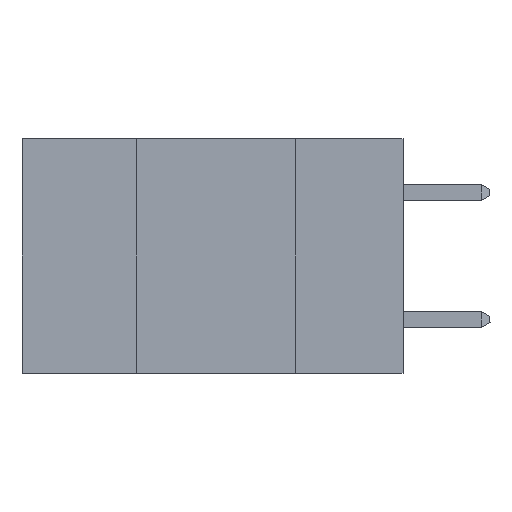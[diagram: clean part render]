
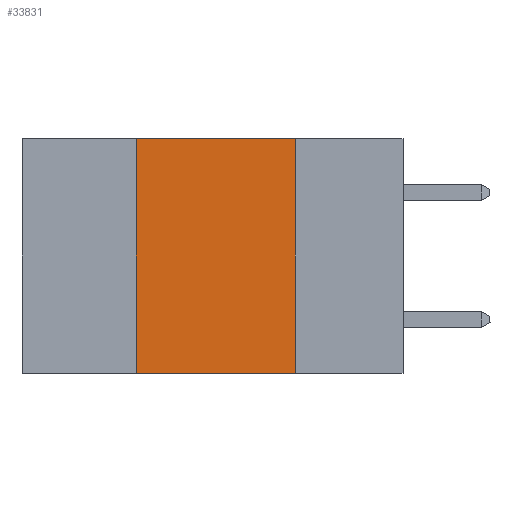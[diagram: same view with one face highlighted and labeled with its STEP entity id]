
A CAD part, left-side view. The second image highlights one B-rep face of the part: STEP entity #33831.
In plain terms, the highlighted planar face has unit normal (-1, 0, 0).
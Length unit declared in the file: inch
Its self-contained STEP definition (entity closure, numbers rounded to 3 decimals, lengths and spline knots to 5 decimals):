
#462 = VERTEX_POINT ( 'NONE', #35231 ) ;
#1846 = VECTOR ( 'NONE', #3232, 39.37008 ) ;
#3232 = DIRECTION ( 'NONE',  ( 0., 0., -1. ) ) ;
#3830 = CARTESIAN_POINT ( 'NONE',  ( 0., 0.17, 0. ) ) ;
#4133 = EDGE_CURVE ( 'NONE', #462, #19122, #25147, .T. ) ;
#5890 = CARTESIAN_POINT ( 'NONE',  ( 0., 0.42, -0.37 ) ) ;
#7984 = CARTESIAN_POINT ( 'NONE',  ( 0., 0.6, 0. ) ) ;
#8055 = EDGE_LOOP ( 'NONE', ( #14364, #28024, #12784, #22752 ) ) ;
#9670 = CARTESIAN_POINT ( 'NONE',  ( 0., 0.42, 0. ) ) ;
#11705 = LINE ( 'NONE', #24902, #14326 ) ;
#12784 = ORIENTED_EDGE ( 'NONE', *, *, #13157, .F. ) ;
#13157 = EDGE_CURVE ( 'NONE', #30707, #26317, #32740, .T. ) ;
#13160 = DIRECTION ( 'NONE',  ( 0., -1., 0. ) ) ;
#14326 = VECTOR ( 'NONE', #19007, 39.37008 ) ;
#14364 = ORIENTED_EDGE ( 'NONE', *, *, #4133, .F. ) ;
#16436 = DIRECTION ( 'NONE',  ( 0., 0., -1. ) ) ;
#16932 = VECTOR ( 'NONE', #34875, 39.37008 ) ;
#17574 = CARTESIAN_POINT ( 'NONE',  ( 0., 0.42, 0. ) ) ;
#19007 = DIRECTION ( 'NONE',  ( 0., -1., 0. ) ) ;
#19122 = VERTEX_POINT ( 'NONE', #19761 ) ;
#19761 = CARTESIAN_POINT ( 'NONE',  ( 0., 0.17, -0.37 ) ) ;
#21827 = AXIS2_PLACEMENT_3D ( 'NONE', #7984, #27585, #16436 ) ;
#22752 = ORIENTED_EDGE ( 'NONE', *, *, #34314, .T. ) ;
#24813 = PLANE ( 'NONE',  #21827 ) ;
#24902 = CARTESIAN_POINT ( 'NONE',  ( 0., 0.6, -0.37 ) ) ;
#25147 = LINE ( 'NONE', #3830, #1846 ) ;
#26317 = VERTEX_POINT ( 'NONE', #17574 ) ;
#27059 = LINE ( 'NONE', #35872, #34124 ) ;
#27585 = DIRECTION ( 'NONE',  ( 1., 0., 0. ) ) ;
#28024 = ORIENTED_EDGE ( 'NONE', *, *, #29425, .F. ) ;
#28367 = FACE_OUTER_BOUND ( 'NONE', #8055, .T. ) ;
#29425 = EDGE_CURVE ( 'NONE', #26317, #462, #27059, .T. ) ;
#30707 = VERTEX_POINT ( 'NONE', #5890 ) ;
#32740 = LINE ( 'NONE', #9670, #16932 ) ;
#33831 = ADVANCED_FACE ( 'NONE', ( #28367 ), #24813, .F. ) ;
#34124 = VECTOR ( 'NONE', #13160, 39.37008 ) ;
#34314 = EDGE_CURVE ( 'NONE', #30707, #19122, #11705, .T. ) ;
#34875 = DIRECTION ( 'NONE',  ( 0., 0., 1. ) ) ;
#35231 = CARTESIAN_POINT ( 'NONE',  ( 0., 0.17, 0. ) ) ;
#35872 = CARTESIAN_POINT ( 'NONE',  ( 0., 0.6, 0. ) ) ;
